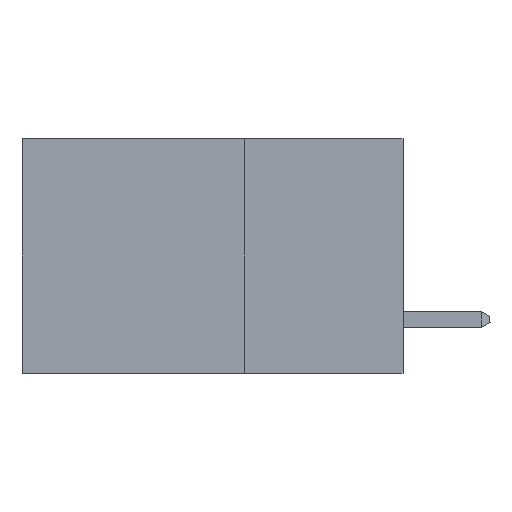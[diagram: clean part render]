
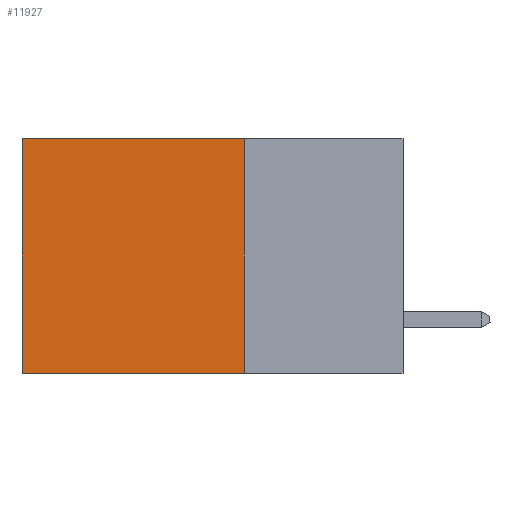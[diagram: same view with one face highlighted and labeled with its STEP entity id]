
A CAD part, left-side view. The second image highlights one B-rep face of the part: STEP entity #11927.
In plain terms, the highlighted planar face has unit normal (-1, 0, 0).
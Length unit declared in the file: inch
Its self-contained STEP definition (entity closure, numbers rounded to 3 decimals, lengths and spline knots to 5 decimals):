
#572 = EDGE_LOOP ( 'NONE', ( #5844, #14242, #9194, #1246 ) ) ;
#681 = CARTESIAN_POINT ( 'NONE',  ( 0.2875, 0.25, 0. ) ) ;
#888 = PLANE ( 'NONE',  #4204 ) ;
#941 = DIRECTION ( 'NONE',  ( 0., 0., -1. ) ) ;
#1246 = ORIENTED_EDGE ( 'NONE', *, *, #6738, .T. ) ;
#1257 = VERTEX_POINT ( 'NONE', #14311 ) ;
#1618 = LINE ( 'NONE', #2670, #3156 ) ;
#2670 = CARTESIAN_POINT ( 'NONE',  ( 0.2875, 0.25, 0. ) ) ;
#2723 = CARTESIAN_POINT ( 'NONE',  ( 0.2875, 0.6, 0. ) ) ;
#2776 = DIRECTION ( 'NONE',  ( 0., 0., -1. ) ) ;
#3156 = VECTOR ( 'NONE', #14743, 39.37008 ) ;
#4204 = AXIS2_PLACEMENT_3D ( 'NONE', #9595, #5924, #941 ) ;
#4295 = EDGE_CURVE ( 'NONE', #11920, #13593, #5421, .T. ) ;
#5421 = LINE ( 'NONE', #9447, #11798 ) ;
#5844 = ORIENTED_EDGE ( 'NONE', *, *, #15360, .T. ) ;
#5924 = DIRECTION ( 'NONE',  ( 1., 0., 0. ) ) ;
#6738 = EDGE_CURVE ( 'NONE', #14184, #1257, #1618, .T. ) ;
#6757 = DIRECTION ( 'NONE',  ( 0., 0., -1. ) ) ;
#6812 = DIRECTION ( 'NONE',  ( 0., 1., 0. ) ) ;
#9194 = ORIENTED_EDGE ( 'NONE', *, *, #15596, .F. ) ;
#9447 = CARTESIAN_POINT ( 'NONE',  ( 0.2875, 0.25, -0.37 ) ) ;
#9545 = CARTESIAN_POINT ( 'NONE',  ( 0.2875, 0.25, -0.37 ) ) ;
#9595 = CARTESIAN_POINT ( 'NONE',  ( 0.2875, 0.25, 0. ) ) ;
#11361 = CARTESIAN_POINT ( 'NONE',  ( 0.2875, 0.25, 0. ) ) ;
#11798 = VECTOR ( 'NONE', #6812, 39.37008 ) ;
#11920 = VERTEX_POINT ( 'NONE', #9545 ) ;
#11927 = ADVANCED_FACE ( 'NONE', ( #15932 ), #888, .F. ) ;
#12035 = VECTOR ( 'NONE', #2776, 39.37008 ) ;
#13593 = VERTEX_POINT ( 'NONE', #16079 ) ;
#13989 = VECTOR ( 'NONE', #6757, 39.37008 ) ;
#14184 = VERTEX_POINT ( 'NONE', #11361 ) ;
#14242 = ORIENTED_EDGE ( 'NONE', *, *, #4295, .F. ) ;
#14311 = CARTESIAN_POINT ( 'NONE',  ( 0.2875, 0.6, 0. ) ) ;
#14743 = DIRECTION ( 'NONE',  ( 0., 1., 0. ) ) ;
#14795 = LINE ( 'NONE', #2723, #12035 ) ;
#15182 = LINE ( 'NONE', #681, #13989 ) ;
#15360 = EDGE_CURVE ( 'NONE', #1257, #13593, #14795, .T. ) ;
#15596 = EDGE_CURVE ( 'NONE', #14184, #11920, #15182, .T. ) ;
#15932 = FACE_OUTER_BOUND ( 'NONE', #572, .T. ) ;
#16079 = CARTESIAN_POINT ( 'NONE',  ( 0.2875, 0.6, -0.37 ) ) ;
